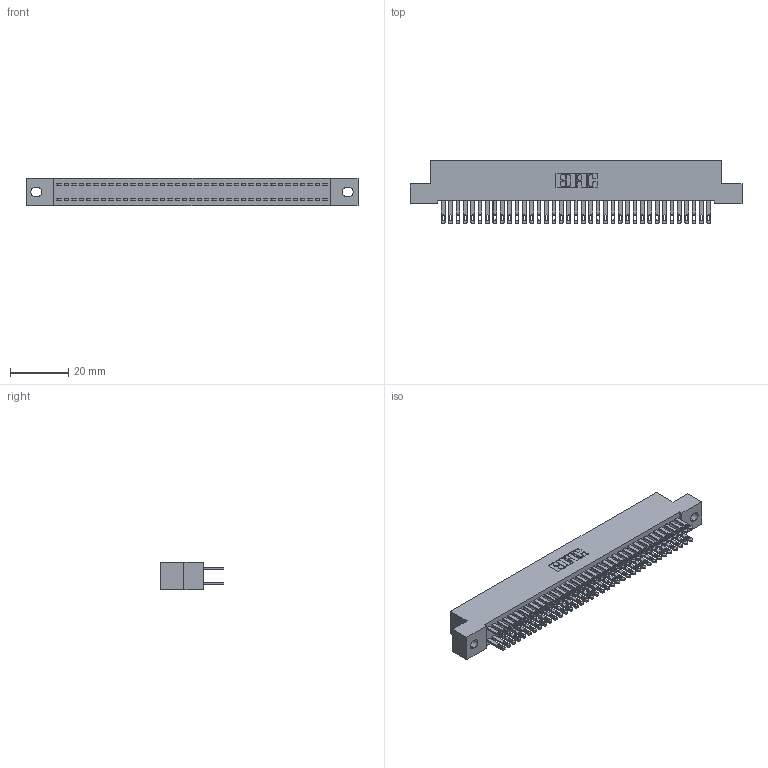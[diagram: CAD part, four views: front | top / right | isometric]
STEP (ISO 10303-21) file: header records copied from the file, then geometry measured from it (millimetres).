
FILE_DESCRIPTION (( 'STEP AP203' ), '1' );
FILE_NAME ('342-074-500-202.STEP', '2019-10-03T16:59:08', ( '' ), ( '' ), 'SwSTEP 2.0', 'SolidWorks 2016', '' );
FILE_SCHEMA (( 'CONFIG_CONTROL_DESIGN' ));
Length unit declared in the file: inch
Products named in the file (3): 342-074-500-202; 342 Part_.128 Slot; 345-292-001_345-293-100
Assembly tree (75 placements, depth 2):
  342-074-500-202
    342 Part_.128 Slot
    345-292-001_345-293-100  x74
Bounding box: 114.3 x 21.85 x 9.4 mm (x, y, z)
Volume: 10420.2 mm3; surface area: 17306.2 mm2
Topology: 75 solids, 75 shells, 3666 faces, 11189 edges, 7458 vertices
Faces by surface type: plane 2290, cylinder 1376
Entity records: 24383 total; most frequent: CARTESIAN_POINT 4046, ORIENTED_EDGE 3982, DIRECTION 3467, EDGE_CURVE 1991, LINE 1859, VECTOR 1859, VERTEX_POINT 1326, AXIS2_PLACEMENT_3D 804
